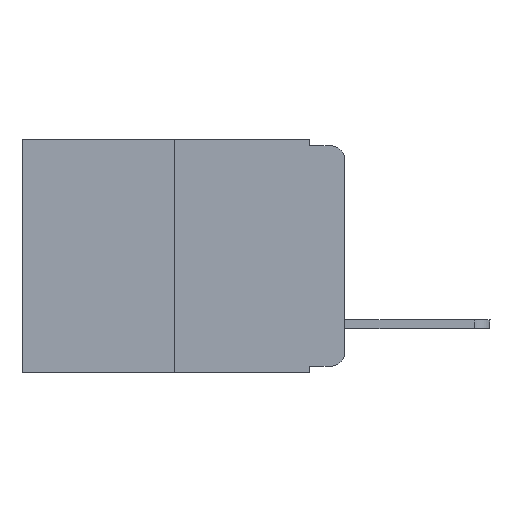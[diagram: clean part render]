
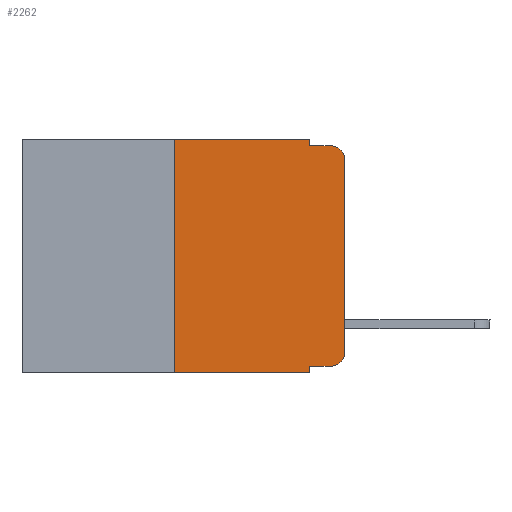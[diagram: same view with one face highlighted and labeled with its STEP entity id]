
A CAD part, left-side view. The second image highlights one B-rep face of the part: STEP entity #2262.
In plain terms, the highlighted planar face has unit normal (-1, 0, 0).
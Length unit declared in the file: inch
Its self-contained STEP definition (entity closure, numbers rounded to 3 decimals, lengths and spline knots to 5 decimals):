
#744 = VECTOR ( 'NONE', #20837, 39.37008 ) ;
#991 = CARTESIAN_POINT ( 'NONE',  ( 0., 0.473, 0. ) ) ;
#1092 = CARTESIAN_POINT ( 'NONE',  ( 0., 0.051, 0. ) ) ;
#1401 = EDGE_CURVE ( 'NONE', #8229, #2186, #5370, .T. ) ;
#2186 = VERTEX_POINT ( 'NONE', #19097 ) ;
#2247 = VERTEX_POINT ( 'NONE', #14644 ) ;
#2262 = ADVANCED_FACE ( 'NONE', ( #2366 ), #5875, .F. ) ;
#2366 = FACE_OUTER_BOUND ( 'NONE', #7187, .T. ) ;
#2944 = CARTESIAN_POINT ( 'NONE',  ( 0., 0.25, 0. ) ) ;
#2988 = EDGE_CURVE ( 'NONE', #21062, #7833, #10709, .T. ) ;
#3643 = CARTESIAN_POINT ( 'NONE',  ( 0., 0.051, 0. ) ) ;
#3694 = AXIS2_PLACEMENT_3D ( 'NONE', #7199, #14120, #8902 ) ;
#4168 = DIRECTION ( 'NONE',  ( 0., -1., 0. ) ) ;
#4420 = CIRCLE ( 'NONE', #3694, 0.02 ) ;
#5370 = LINE ( 'NONE', #15732, #13196 ) ;
#5527 = EDGE_CURVE ( 'NONE', #2186, #9970, #4420, .T. ) ;
#5875 = PLANE ( 'NONE',  #17380 ) ;
#5958 = CARTESIAN_POINT ( 'NONE',  ( 0., 0.051, -0.333 ) ) ;
#6502 = EDGE_CURVE ( 'NONE', #13124, #22437, #10774, .T. ) ;
#6613 = ORIENTED_EDGE ( 'NONE', *, *, #1401, .T. ) ;
#6649 = VECTOR ( 'NONE', #4168, 39.37008 ) ;
#6847 = DIRECTION ( 'NONE',  ( 0., 0., -1. ) ) ;
#7019 = ORIENTED_EDGE ( 'NONE', *, *, #22488, .T. ) ;
#7187 = EDGE_LOOP ( 'NONE', ( #6613, #9083, #12049, #11771, #12834, #12180, #13268, #16695, #12534, #7019 ) ) ;
#7199 = CARTESIAN_POINT ( 'NONE',  ( 0., 0.02, -0.03 ) ) ;
#7833 = VERTEX_POINT ( 'NONE', #11325 ) ;
#7920 = EDGE_CURVE ( 'NONE', #22437, #2247, #22024, .T. ) ;
#8057 = EDGE_CURVE ( 'NONE', #21062, #13124, #22361, .T. ) ;
#8229 = VERTEX_POINT ( 'NONE', #17781 ) ;
#8548 = CARTESIAN_POINT ( 'NONE',  ( 0., 0.02, -0.313 ) ) ;
#8707 = DIRECTION ( 'NONE',  ( 0., 0., 1. ) ) ;
#8902 = DIRECTION ( 'NONE',  ( 0., 0., -1. ) ) ;
#9083 = ORIENTED_EDGE ( 'NONE', *, *, #5527, .T. ) ;
#9209 = CIRCLE ( 'NONE', #12104, 0.02 ) ;
#9261 = VECTOR ( 'NONE', #17853, 39.37008 ) ;
#9459 = EDGE_CURVE ( 'NONE', #17444, #7833, #11637, .T. ) ;
#9970 = VERTEX_POINT ( 'NONE', #10657 ) ;
#10322 = VECTOR ( 'NONE', #14857, 39.37008 ) ;
#10657 = CARTESIAN_POINT ( 'NONE',  ( 0., 0.02, -0.01 ) ) ;
#10709 = LINE ( 'NONE', #12522, #9261 ) ;
#10774 = LINE ( 'NONE', #12700, #6649 ) ;
#10848 = VECTOR ( 'NONE', #14392, 39.37008 ) ;
#11325 = CARTESIAN_POINT ( 'NONE',  ( 0., 0.051, -0.343 ) ) ;
#11384 = CARTESIAN_POINT ( 'NONE',  ( 0., 0.25, -0.343 ) ) ;
#11637 = LINE ( 'NONE', #22102, #16199 ) ;
#11771 = ORIENTED_EDGE ( 'NONE', *, *, #7920, .F. ) ;
#12049 = ORIENTED_EDGE ( 'NONE', *, *, #17949, .F. ) ;
#12104 = AXIS2_PLACEMENT_3D ( 'NONE', #8548, #15481, #6847 ) ;
#12180 = ORIENTED_EDGE ( 'NONE', *, *, #8057, .F. ) ;
#12522 = CARTESIAN_POINT ( 'NONE',  ( 0., 0.473, -0.343 ) ) ;
#12534 = ORIENTED_EDGE ( 'NONE', *, *, #13821, .T. ) ;
#12545 = DIRECTION ( 'NONE',  ( 0., 0., 1. ) ) ;
#12700 = CARTESIAN_POINT ( 'NONE',  ( 0., 0.473, 0. ) ) ;
#12834 = ORIENTED_EDGE ( 'NONE', *, *, #6502, .F. ) ;
#13004 = DIRECTION ( 'NONE',  ( 0., 0., -1. ) ) ;
#13124 = VERTEX_POINT ( 'NONE', #2944 ) ;
#13196 = VECTOR ( 'NONE', #12545, 39.37008 ) ;
#13268 = ORIENTED_EDGE ( 'NONE', *, *, #2988, .T. ) ;
#13598 = CARTESIAN_POINT ( 'NONE',  ( 0., 0.25, 0. ) ) ;
#13821 = EDGE_CURVE ( 'NONE', #17444, #16568, #14161, .T. ) ;
#14120 = DIRECTION ( 'NONE',  ( -1., 0., 0. ) ) ;
#14161 = LINE ( 'NONE', #5958, #10848 ) ;
#14392 = DIRECTION ( 'NONE',  ( 0., -1., 0. ) ) ;
#14644 = CARTESIAN_POINT ( 'NONE',  ( 0., 0.051, -0.01 ) ) ;
#14857 = DIRECTION ( 'NONE',  ( 0., 0., -1. ) ) ;
#15208 = CARTESIAN_POINT ( 'NONE',  ( 0., 0.051, -0.333 ) ) ;
#15481 = DIRECTION ( 'NONE',  ( -1., 0., 0. ) ) ;
#15732 = CARTESIAN_POINT ( 'NONE',  ( 0., 0., 0. ) ) ;
#16199 = VECTOR ( 'NONE', #13004, 39.37008 ) ;
#16236 = DIRECTION ( 'NONE',  ( 0., 0., -1. ) ) ;
#16568 = VERTEX_POINT ( 'NONE', #22490 ) ;
#16695 = ORIENTED_EDGE ( 'NONE', *, *, #9459, .F. ) ;
#17066 = CARTESIAN_POINT ( 'NONE',  ( 0., 0.051, -0.01 ) ) ;
#17380 = AXIS2_PLACEMENT_3D ( 'NONE', #991, #21798, #16236 ) ;
#17444 = VERTEX_POINT ( 'NONE', #15208 ) ;
#17781 = CARTESIAN_POINT ( 'NONE',  ( 0., 0., -0.313 ) ) ;
#17853 = DIRECTION ( 'NONE',  ( 0., -1., 0. ) ) ;
#17949 = EDGE_CURVE ( 'NONE', #2247, #9970, #18790, .T. ) ;
#18790 = LINE ( 'NONE', #17066, #744 ) ;
#19097 = CARTESIAN_POINT ( 'NONE',  ( 0., 0., -0.03 ) ) ;
#20837 = DIRECTION ( 'NONE',  ( 0., -1., 0. ) ) ;
#21062 = VERTEX_POINT ( 'NONE', #11384 ) ;
#21798 = DIRECTION ( 'NONE',  ( 1., 0., 0. ) ) ;
#21956 = VECTOR ( 'NONE', #8707, 39.37008 ) ;
#22024 = LINE ( 'NONE', #1092, #10322 ) ;
#22102 = CARTESIAN_POINT ( 'NONE',  ( 0., 0.051, 0. ) ) ;
#22361 = LINE ( 'NONE', #13598, #21956 ) ;
#22437 = VERTEX_POINT ( 'NONE', #3643 ) ;
#22488 = EDGE_CURVE ( 'NONE', #16568, #8229, #9209, .T. ) ;
#22490 = CARTESIAN_POINT ( 'NONE',  ( 0., 0.02, -0.333 ) ) ;
